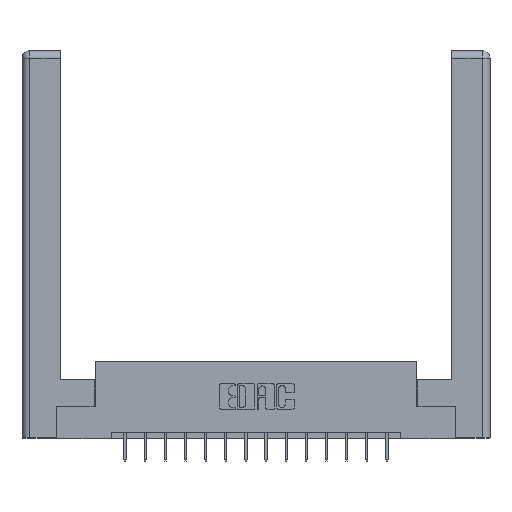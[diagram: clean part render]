
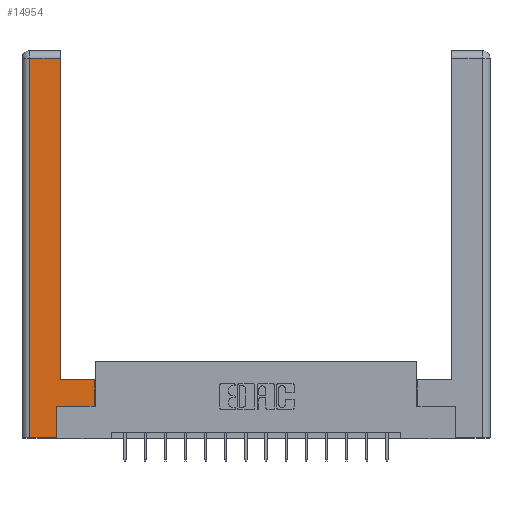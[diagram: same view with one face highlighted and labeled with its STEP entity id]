
A CAD part, top view. The second image highlights one B-rep face of the part: STEP entity #14954.
In plain terms, the highlighted planar face has unit normal (0, 0, 1).
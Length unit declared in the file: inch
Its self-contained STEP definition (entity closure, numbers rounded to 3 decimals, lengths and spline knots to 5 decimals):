
#16 = EDGE_CURVE ( 'NONE', #15831, #13393, #12390, .T. ) ;
#32 = FACE_OUTER_BOUND ( 'NONE', #4374, .T. ) ;
#153 = VECTOR ( 'NONE', #1479, 39.37008 ) ;
#159 = ORIENTED_EDGE ( 'NONE', *, *, #336, .T. ) ;
#336 = EDGE_CURVE ( 'NONE', #4619, #13469, #5516, .T. ) ;
#560 = AXIS2_PLACEMENT_3D ( 'NONE', #11586, #6243, #3661 ) ;
#598 = CARTESIAN_POINT ( 'NONE',  ( 0.295, 0.45, 0. ) ) ;
#618 = CARTESIAN_POINT ( 'NONE',  ( 0.565, 0.245, 0. ) ) ;
#679 = LINE ( 'NONE', #14635, #1287 ) ;
#702 = VECTOR ( 'NONE', #3377, 39.37008 ) ;
#838 = LINE ( 'NONE', #12019, #3982 ) ;
#1287 = VECTOR ( 'NONE', #15795, 39.37008 ) ;
#1479 = DIRECTION ( 'NONE',  ( 1., 0., 0. ) ) ;
#1702 = CARTESIAN_POINT ( 'NONE',  ( 0.265, 0.245, 0. ) ) ;
#1819 = DIRECTION ( 'NONE',  ( -1., 0., 0. ) ) ;
#2319 = DIRECTION ( 'NONE',  ( 0., -1., 0. ) ) ;
#2741 = ORIENTED_EDGE ( 'NONE', *, *, #17031, .T. ) ;
#3262 = CARTESIAN_POINT ( 'NONE',  ( 0.0615, 0., 0. ) ) ;
#3377 = DIRECTION ( 'NONE',  ( 0., 1., 0. ) ) ;
#3661 = DIRECTION ( 'NONE',  ( -1., 0., 0. ) ) ;
#3755 = DIRECTION ( 'NONE',  ( 0., 1., 0. ) ) ;
#3982 = VECTOR ( 'NONE', #13383, 39.37008 ) ;
#4374 = EDGE_LOOP ( 'NONE', ( #159, #12667, #6477, #8226, #6000, #2741, #6816, #13423 ) ) ;
#4619 = VERTEX_POINT ( 'NONE', #13330 ) ;
#4918 = EDGE_CURVE ( 'NONE', #10521, #4995, #11276, .T. ) ;
#4923 = CARTESIAN_POINT ( 'NONE',  ( 0.0615, 2.94, 0. ) ) ;
#4995 = VERTEX_POINT ( 'NONE', #6439 ) ;
#5516 = LINE ( 'NONE', #6466, #16532 ) ;
#5947 = CARTESIAN_POINT ( 'NONE',  ( 0.265, 0., 0. ) ) ;
#5974 = EDGE_CURVE ( 'NONE', #13469, #14929, #679, .T. ) ;
#6000 = ORIENTED_EDGE ( 'NONE', *, *, #7025, .T. ) ;
#6243 = DIRECTION ( 'NONE',  ( 0., 0., -1. ) ) ;
#6439 = CARTESIAN_POINT ( 'NONE',  ( 0.565, 0.45, 0. ) ) ;
#6466 = CARTESIAN_POINT ( 'NONE',  ( 0.295, 3., 0. ) ) ;
#6477 = ORIENTED_EDGE ( 'NONE', *, *, #12085, .T. ) ;
#6633 = CARTESIAN_POINT ( 'NONE',  ( 0.265, 0., 0. ) ) ;
#6816 = ORIENTED_EDGE ( 'NONE', *, *, #4918, .T. ) ;
#7025 = EDGE_CURVE ( 'NONE', #13393, #14966, #838, .T. ) ;
#7328 = VECTOR ( 'NONE', #13636, 39.37008 ) ;
#7585 = CARTESIAN_POINT ( 'NONE',  ( 0.565, 0.45, 0. ) ) ;
#8049 = LINE ( 'NONE', #13118, #8684 ) ;
#8194 = LINE ( 'NONE', #598, #12764 ) ;
#8226 = ORIENTED_EDGE ( 'NONE', *, *, #16, .T. ) ;
#8684 = VECTOR ( 'NONE', #2319, 39.37008 ) ;
#9679 = CARTESIAN_POINT ( 'NONE',  ( 0.565, 0.245, 0. ) ) ;
#10220 = CARTESIAN_POINT ( 'NONE',  ( 0.295, 2.94, 0. ) ) ;
#10521 = VERTEX_POINT ( 'NONE', #9679 ) ;
#10838 = LINE ( 'NONE', #618, #7328 ) ;
#11276 = LINE ( 'NONE', #7585, #702 ) ;
#11586 = CARTESIAN_POINT ( 'NONE',  ( 0., 0., 0. ) ) ;
#12019 = CARTESIAN_POINT ( 'NONE',  ( 0.265, 0.245, 0. ) ) ;
#12085 = EDGE_CURVE ( 'NONE', #14929, #15831, #8049, .T. ) ;
#12390 = LINE ( 'NONE', #6633, #153 ) ;
#12667 = ORIENTED_EDGE ( 'NONE', *, *, #5974, .T. ) ;
#12764 = VECTOR ( 'NONE', #1819, 39.37008 ) ;
#13118 = CARTESIAN_POINT ( 'NONE',  ( 0.0615, 0., 0. ) ) ;
#13330 = CARTESIAN_POINT ( 'NONE',  ( 0.295, 0.45, 0. ) ) ;
#13383 = DIRECTION ( 'NONE',  ( 0., 1., 0. ) ) ;
#13393 = VERTEX_POINT ( 'NONE', #5947 ) ;
#13423 = ORIENTED_EDGE ( 'NONE', *, *, #13672, .T. ) ;
#13469 = VERTEX_POINT ( 'NONE', #10220 ) ;
#13636 = DIRECTION ( 'NONE',  ( 1., 0., 0. ) ) ;
#13672 = EDGE_CURVE ( 'NONE', #4995, #4619, #8194, .T. ) ;
#14188 = PLANE ( 'NONE',  #560 ) ;
#14635 = CARTESIAN_POINT ( 'NONE',  ( 0.0615, 2.94, 0. ) ) ;
#14929 = VERTEX_POINT ( 'NONE', #4923 ) ;
#14954 = ADVANCED_FACE ( 'NONE', ( #32 ), #14188, .F. ) ;
#14966 = VERTEX_POINT ( 'NONE', #1702 ) ;
#15795 = DIRECTION ( 'NONE',  ( -1., 0., 0. ) ) ;
#15831 = VERTEX_POINT ( 'NONE', #3262 ) ;
#16532 = VECTOR ( 'NONE', #3755, 39.37008 ) ;
#17031 = EDGE_CURVE ( 'NONE', #14966, #10521, #10838, .T. ) ;
